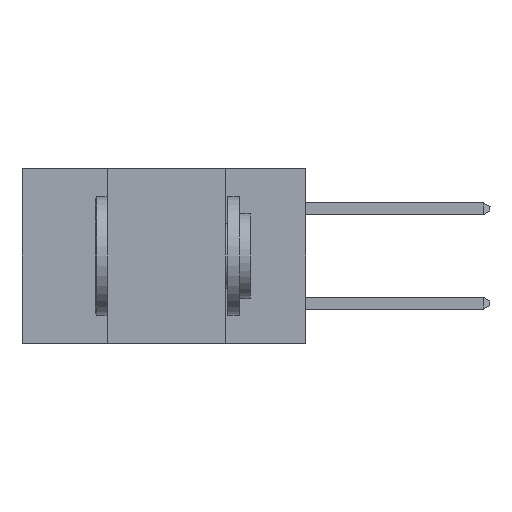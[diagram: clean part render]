
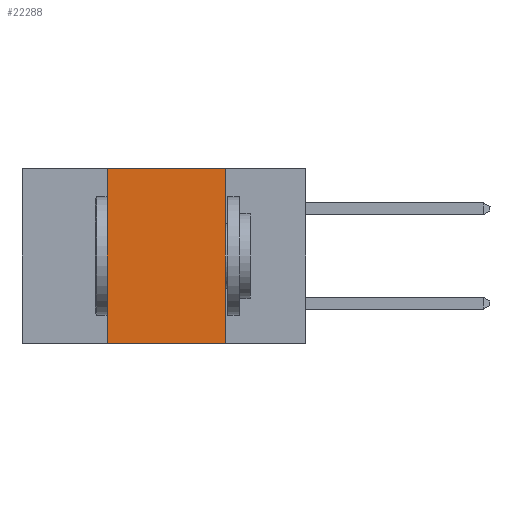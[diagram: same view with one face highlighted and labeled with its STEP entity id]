
A CAD part, left-side view. The second image highlights one B-rep face of the part: STEP entity #22288.
In plain terms, the highlighted planar face has unit normal (-1, 0, 0).
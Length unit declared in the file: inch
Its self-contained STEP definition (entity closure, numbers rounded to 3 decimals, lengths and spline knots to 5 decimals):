
#30 = ORIENTED_EDGE ( 'NONE', *, *, #19532, .F. ) ;
#429 = ORIENTED_EDGE ( 'NONE', *, *, #24611, .T. ) ;
#719 = VERTEX_POINT ( 'NONE', #17338 ) ;
#1612 = EDGE_CURVE ( 'NONE', #719, #16845, #28548, .T. ) ;
#1619 = DIRECTION ( 'NONE',  ( 0., 0., -1. ) ) ;
#4572 = EDGE_LOOP ( 'NONE', ( #7891, #30, #27775, #429 ) ) ;
#6618 = CARTESIAN_POINT ( 'NONE',  ( 0., 0.6, 0. ) ) ;
#7891 = ORIENTED_EDGE ( 'NONE', *, *, #19723, .F. ) ;
#8791 = DIRECTION ( 'NONE',  ( 0., 0., 1. ) ) ;
#9915 = DIRECTION ( 'NONE',  ( 0., 0., -1. ) ) ;
#10977 = VECTOR ( 'NONE', #19642, 39.37008 ) ;
#12550 = AXIS2_PLACEMENT_3D ( 'NONE', #6618, #16826, #1619 ) ;
#12692 = FACE_OUTER_BOUND ( 'NONE', #4572, .T. ) ;
#14260 = DIRECTION ( 'NONE',  ( 0., -1., 0. ) ) ;
#15626 = VECTOR ( 'NONE', #14260, 39.37008 ) ;
#16453 = LINE ( 'NONE', #19388, #15626 ) ;
#16826 = DIRECTION ( 'NONE',  ( 1., 0., 0. ) ) ;
#16845 = VERTEX_POINT ( 'NONE', #18943 ) ;
#16996 = LINE ( 'NONE', #32228, #10977 ) ;
#17338 = CARTESIAN_POINT ( 'NONE',  ( 0., 0.42, -0.37 ) ) ;
#18577 = VERTEX_POINT ( 'NONE', #20762 ) ;
#18943 = CARTESIAN_POINT ( 'NONE',  ( 0., 0.42, 0. ) ) ;
#19388 = CARTESIAN_POINT ( 'NONE',  ( 0., 0.6, 0. ) ) ;
#19532 = EDGE_CURVE ( 'NONE', #16845, #18577, #16453, .T. ) ;
#19642 = DIRECTION ( 'NONE',  ( 0., -1., 0. ) ) ;
#19723 = EDGE_CURVE ( 'NONE', #18577, #29594, #24381, .T. ) ;
#20762 = CARTESIAN_POINT ( 'NONE',  ( 0., 0.17, 0. ) ) ;
#22288 = ADVANCED_FACE ( 'NONE', ( #12692 ), #31950, .F. ) ;
#22617 = CARTESIAN_POINT ( 'NONE',  ( 0., 0.17, 0. ) ) ;
#22785 = VECTOR ( 'NONE', #9915, 39.37008 ) ;
#24381 = LINE ( 'NONE', #22617, #22785 ) ;
#24611 = EDGE_CURVE ( 'NONE', #719, #29594, #16996, .T. ) ;
#27775 = ORIENTED_EDGE ( 'NONE', *, *, #1612, .F. ) ;
#28548 = LINE ( 'NONE', #30029, #29345 ) ;
#29345 = VECTOR ( 'NONE', #8791, 39.37008 ) ;
#29594 = VERTEX_POINT ( 'NONE', #31536 ) ;
#30029 = CARTESIAN_POINT ( 'NONE',  ( 0., 0.42, 0. ) ) ;
#31536 = CARTESIAN_POINT ( 'NONE',  ( 0., 0.17, -0.37 ) ) ;
#31950 = PLANE ( 'NONE',  #12550 ) ;
#32228 = CARTESIAN_POINT ( 'NONE',  ( 0., 0.6, -0.37 ) ) ;
